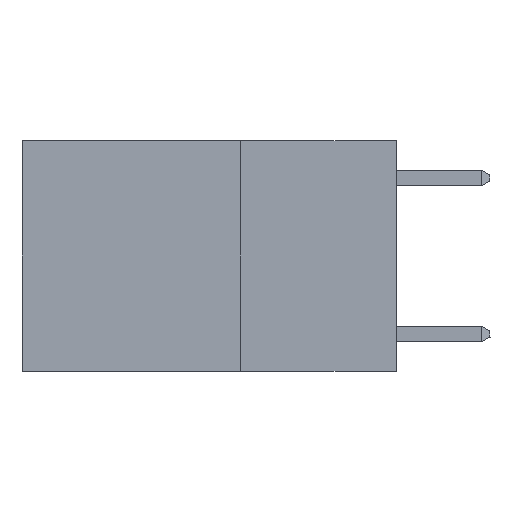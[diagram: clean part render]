
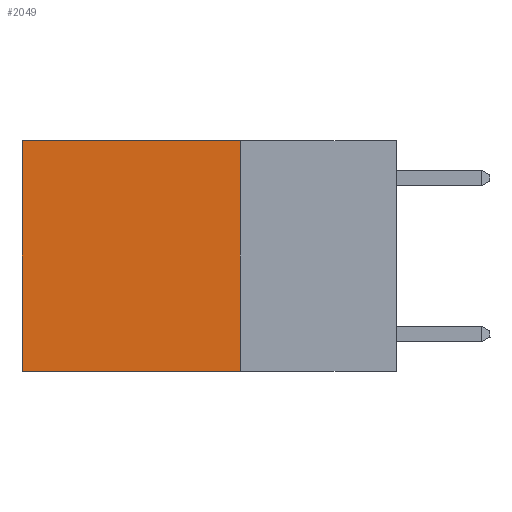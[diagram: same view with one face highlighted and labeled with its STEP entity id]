
A CAD part, left-side view. The second image highlights one B-rep face of the part: STEP entity #2049.
In plain terms, the highlighted planar face has unit normal (-1, 0, 0).
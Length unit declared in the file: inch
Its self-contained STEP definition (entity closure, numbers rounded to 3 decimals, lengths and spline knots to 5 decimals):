
#644 = VERTEX_POINT ( 'NONE', #13248 ) ;
#1077 = DIRECTION ( 'NONE',  ( 0., 0., -1. ) ) ;
#2049 = ADVANCED_FACE ( 'NONE', ( #2351 ), #4255, .F. ) ;
#2351 = FACE_OUTER_BOUND ( 'NONE', #17043, .T. ) ;
#3041 = ORIENTED_EDGE ( 'NONE', *, *, #16700, .T. ) ;
#3317 = DIRECTION ( 'NONE',  ( 0., 0., -1. ) ) ;
#3348 = DIRECTION ( 'NONE',  ( 1., 0., 0. ) ) ;
#3627 = ORIENTED_EDGE ( 'NONE', *, *, #24136, .F. ) ;
#3740 = CARTESIAN_POINT ( 'NONE',  ( 0.2625, 0.25, 0. ) ) ;
#4131 = LINE ( 'NONE', #17142, #18803 ) ;
#4255 = PLANE ( 'NONE',  #17089 ) ;
#6066 = VECTOR ( 'NONE', #17835, 39.37008 ) ;
#6122 = CARTESIAN_POINT ( 'NONE',  ( 0.2625, 0.25, -0.37 ) ) ;
#6721 = LINE ( 'NONE', #15978, #6066 ) ;
#7061 = EDGE_CURVE ( 'NONE', #644, #7619, #6721, .T. ) ;
#7619 = VERTEX_POINT ( 'NONE', #10528 ) ;
#9230 = CARTESIAN_POINT ( 'NONE',  ( 0.2625, 0.25, -0.37 ) ) ;
#9625 = VECTOR ( 'NONE', #22268, 39.37008 ) ;
#10528 = CARTESIAN_POINT ( 'NONE',  ( 0.2625, 0.6, 0. ) ) ;
#10690 = EDGE_CURVE ( 'NONE', #17632, #20217, #23833, .T. ) ;
#13248 = CARTESIAN_POINT ( 'NONE',  ( 0.2625, 0.25, 0. ) ) ;
#15978 = CARTESIAN_POINT ( 'NONE',  ( 0.2625, 0.25, 0. ) ) ;
#16031 = VECTOR ( 'NONE', #1077, 39.37008 ) ;
#16700 = EDGE_CURVE ( 'NONE', #7619, #20217, #4131, .T. ) ;
#17043 = EDGE_LOOP ( 'NONE', ( #3041, #21908, #3627, #18945 ) ) ;
#17089 = AXIS2_PLACEMENT_3D ( 'NONE', #3740, #3348, #3317 ) ;
#17142 = CARTESIAN_POINT ( 'NONE',  ( 0.2625, 0.6, 0. ) ) ;
#17632 = VERTEX_POINT ( 'NONE', #6122 ) ;
#17770 = LINE ( 'NONE', #22207, #16031 ) ;
#17835 = DIRECTION ( 'NONE',  ( 0., 1., 0. ) ) ;
#18803 = VECTOR ( 'NONE', #18974, 39.37008 ) ;
#18945 = ORIENTED_EDGE ( 'NONE', *, *, #7061, .T. ) ;
#18974 = DIRECTION ( 'NONE',  ( 0., 0., -1. ) ) ;
#19313 = CARTESIAN_POINT ( 'NONE',  ( 0.2625, 0.6, -0.37 ) ) ;
#20217 = VERTEX_POINT ( 'NONE', #19313 ) ;
#21908 = ORIENTED_EDGE ( 'NONE', *, *, #10690, .F. ) ;
#22207 = CARTESIAN_POINT ( 'NONE',  ( 0.2625, 0.25, 0. ) ) ;
#22268 = DIRECTION ( 'NONE',  ( 0., 1., 0. ) ) ;
#23833 = LINE ( 'NONE', #9230, #9625 ) ;
#24136 = EDGE_CURVE ( 'NONE', #644, #17632, #17770, .T. ) ;
